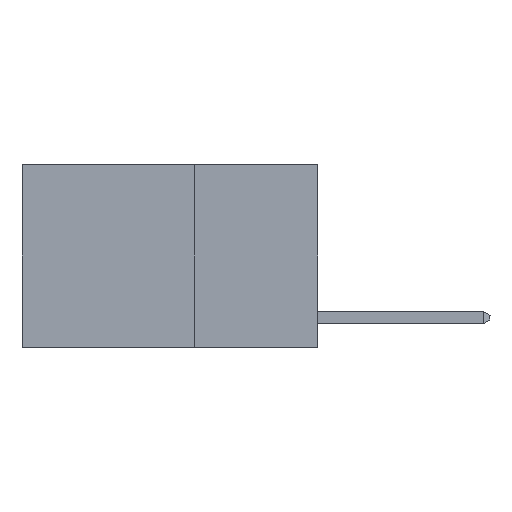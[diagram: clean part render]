
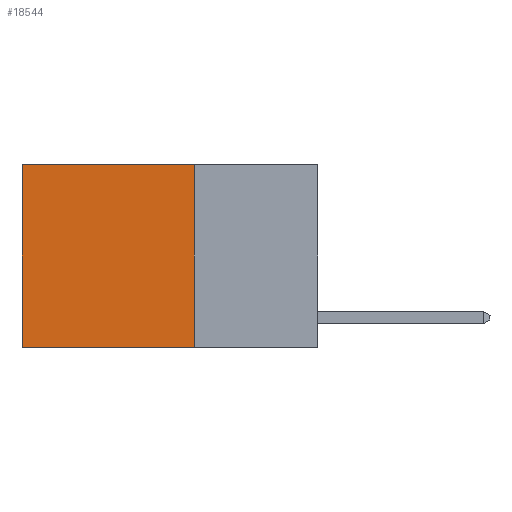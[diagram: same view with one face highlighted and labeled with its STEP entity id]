
A CAD part, left-side view. The second image highlights one B-rep face of the part: STEP entity #18544.
In plain terms, the highlighted planar face has unit normal (-1, 0, 0).
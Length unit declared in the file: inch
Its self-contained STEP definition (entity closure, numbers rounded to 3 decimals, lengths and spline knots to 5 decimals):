
#155 = PLANE ( 'NONE',  #14996 ) ;
#627 = EDGE_CURVE ( 'NONE', #24936, #11274, #12678, .T. ) ;
#1243 = LINE ( 'NONE', #24002, #16258 ) ;
#1641 = EDGE_CURVE ( 'NONE', #24936, #5031, #9551, .T. ) ;
#2572 = DIRECTION ( 'NONE',  ( 0., 0., -1. ) ) ;
#2832 = LINE ( 'NONE', #14076, #12641 ) ;
#4133 = DIRECTION ( 'NONE',  ( 1., 0., 0. ) ) ;
#4466 = ORIENTED_EDGE ( 'NONE', *, *, #12572, .F. ) ;
#4625 = ORIENTED_EDGE ( 'NONE', *, *, #1641, .F. ) ;
#4800 = ORIENTED_EDGE ( 'NONE', *, *, #13282, .T. ) ;
#5031 = VERTEX_POINT ( 'NONE', #17027 ) ;
#5541 = CARTESIAN_POINT ( 'NONE',  ( 0.2625, 0.6, -0.37 ) ) ;
#5623 = DIRECTION ( 'NONE',  ( 0., 0., -1. ) ) ;
#6163 = CARTESIAN_POINT ( 'NONE',  ( 0.2625, 0.25, 0. ) ) ;
#7374 = ORIENTED_EDGE ( 'NONE', *, *, #627, .T. ) ;
#9551 = LINE ( 'NONE', #11512, #14757 ) ;
#11274 = VERTEX_POINT ( 'NONE', #22660 ) ;
#11512 = CARTESIAN_POINT ( 'NONE',  ( 0.2625, 0.25, 0. ) ) ;
#12572 = EDGE_CURVE ( 'NONE', #5031, #14327, #2832, .T. ) ;
#12641 = VECTOR ( 'NONE', #21905, 39.37008 ) ;
#12678 = LINE ( 'NONE', #6163, #22432 ) ;
#13282 = EDGE_CURVE ( 'NONE', #11274, #14327, #1243, .T. ) ;
#14076 = CARTESIAN_POINT ( 'NONE',  ( 0.2625, 0.25, -0.37 ) ) ;
#14327 = VERTEX_POINT ( 'NONE', #5541 ) ;
#14757 = VECTOR ( 'NONE', #5623, 39.37008 ) ;
#14996 = AXIS2_PLACEMENT_3D ( 'NONE', #15830, #4133, #17783 ) ;
#15830 = CARTESIAN_POINT ( 'NONE',  ( 0.2625, 0.25, 0. ) ) ;
#16258 = VECTOR ( 'NONE', #2572, 39.37008 ) ;
#17027 = CARTESIAN_POINT ( 'NONE',  ( 0.2625, 0.25, -0.37 ) ) ;
#17783 = DIRECTION ( 'NONE',  ( 0., 0., -1. ) ) ;
#18544 = ADVANCED_FACE ( 'NONE', ( #23648 ), #155, .F. ) ;
#20135 = EDGE_LOOP ( 'NONE', ( #4800, #4466, #4625, #7374 ) ) ;
#21271 = CARTESIAN_POINT ( 'NONE',  ( 0.2625, 0.25, 0. ) ) ;
#21759 = DIRECTION ( 'NONE',  ( 0., 1., 0. ) ) ;
#21905 = DIRECTION ( 'NONE',  ( 0., 1., 0. ) ) ;
#22432 = VECTOR ( 'NONE', #21759, 39.37008 ) ;
#22660 = CARTESIAN_POINT ( 'NONE',  ( 0.2625, 0.6, 0. ) ) ;
#23648 = FACE_OUTER_BOUND ( 'NONE', #20135, .T. ) ;
#24002 = CARTESIAN_POINT ( 'NONE',  ( 0.2625, 0.6, 0. ) ) ;
#24936 = VERTEX_POINT ( 'NONE', #21271 ) ;
